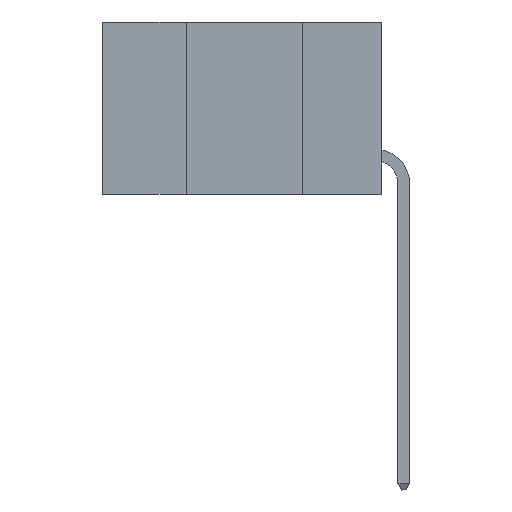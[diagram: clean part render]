
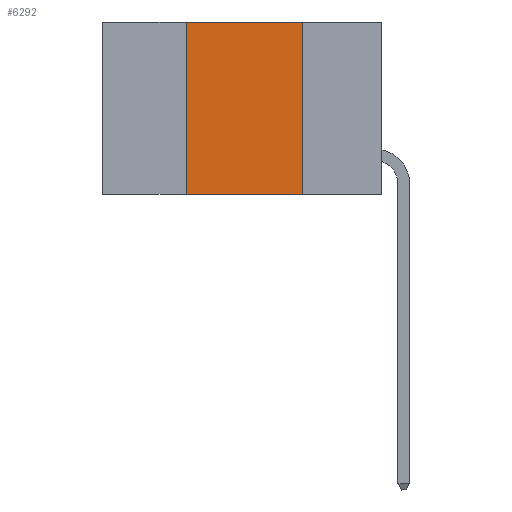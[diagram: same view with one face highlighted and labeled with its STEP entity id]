
A CAD part, left-side view. The second image highlights one B-rep face of the part: STEP entity #6292.
In plain terms, the highlighted planar face has unit normal (-1, 0, 0).
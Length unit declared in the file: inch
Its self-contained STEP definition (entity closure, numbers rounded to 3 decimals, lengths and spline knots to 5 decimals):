
#497 = VECTOR ( 'NONE', #14856, 39.37008 ) ;
#1791 = EDGE_CURVE ( 'NONE', #16573, #9311, #3719, .T. ) ;
#1797 = EDGE_CURVE ( 'NONE', #6507, #16573, #10095, .T. ) ;
#1972 = LINE ( 'NONE', #14960, #5388 ) ;
#2765 = ORIENTED_EDGE ( 'NONE', *, *, #15752, .T. ) ;
#3719 = LINE ( 'NONE', #11395, #8612 ) ;
#4906 = ORIENTED_EDGE ( 'NONE', *, *, #10242, .F. ) ;
#5388 = VECTOR ( 'NONE', #10883, 39.37008 ) ;
#5821 = CARTESIAN_POINT ( 'NONE',  ( 0., 0.42, -0.37 ) ) ;
#6292 = ADVANCED_FACE ( 'NONE', ( #12705 ), #9310, .F. ) ;
#6507 = VERTEX_POINT ( 'NONE', #8518 ) ;
#7307 = VECTOR ( 'NONE', #15167, 39.37008 ) ;
#8518 = CARTESIAN_POINT ( 'NONE',  ( 0., 0.42, 0. ) ) ;
#8612 = VECTOR ( 'NONE', #14639, 39.37008 ) ;
#9191 = DIRECTION ( 'NONE',  ( 0., 0., -1. ) ) ;
#9296 = VERTEX_POINT ( 'NONE', #5821 ) ;
#9310 = PLANE ( 'NONE',  #13090 ) ;
#9311 = VERTEX_POINT ( 'NONE', #15197 ) ;
#10095 = LINE ( 'NONE', #14691, #497 ) ;
#10242 = EDGE_CURVE ( 'NONE', #9296, #6507, #11586, .T. ) ;
#10859 = EDGE_LOOP ( 'NONE', ( #12509, #11212, #4906, #2765 ) ) ;
#10883 = DIRECTION ( 'NONE',  ( 0., -1., 0. ) ) ;
#11212 = ORIENTED_EDGE ( 'NONE', *, *, #1797, .F. ) ;
#11395 = CARTESIAN_POINT ( 'NONE',  ( 0., 0.17, 0. ) ) ;
#11586 = LINE ( 'NONE', #13693, #7307 ) ;
#11977 = DIRECTION ( 'NONE',  ( 1., 0., 0. ) ) ;
#12509 = ORIENTED_EDGE ( 'NONE', *, *, #1791, .F. ) ;
#12705 = FACE_OUTER_BOUND ( 'NONE', #10859, .T. ) ;
#13090 = AXIS2_PLACEMENT_3D ( 'NONE', #17387, #11977, #9191 ) ;
#13693 = CARTESIAN_POINT ( 'NONE',  ( 0., 0.42, 0. ) ) ;
#14639 = DIRECTION ( 'NONE',  ( 0., 0., -1. ) ) ;
#14691 = CARTESIAN_POINT ( 'NONE',  ( 0., 0.6, 0. ) ) ;
#14856 = DIRECTION ( 'NONE',  ( 0., -1., 0. ) ) ;
#14960 = CARTESIAN_POINT ( 'NONE',  ( 0., 0.6, -0.37 ) ) ;
#15167 = DIRECTION ( 'NONE',  ( 0., 0., 1. ) ) ;
#15197 = CARTESIAN_POINT ( 'NONE',  ( 0., 0.17, -0.37 ) ) ;
#15752 = EDGE_CURVE ( 'NONE', #9296, #9311, #1972, .T. ) ;
#16573 = VERTEX_POINT ( 'NONE', #16712 ) ;
#16712 = CARTESIAN_POINT ( 'NONE',  ( 0., 0.17, 0. ) ) ;
#17387 = CARTESIAN_POINT ( 'NONE',  ( 0., 0.6, 0. ) ) ;
